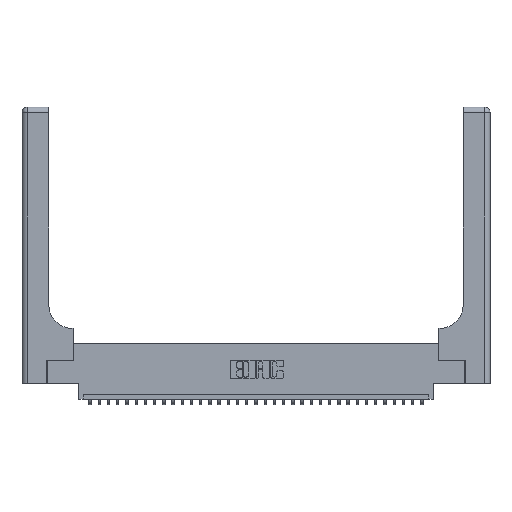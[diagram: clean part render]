
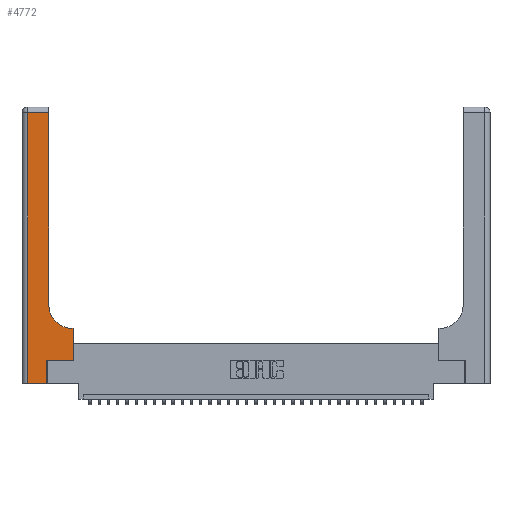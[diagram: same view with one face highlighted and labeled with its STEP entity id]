
A CAD part, top view. The second image highlights one B-rep face of the part: STEP entity #4772.
In plain terms, the highlighted planar face has unit normal (0, 0, 1).
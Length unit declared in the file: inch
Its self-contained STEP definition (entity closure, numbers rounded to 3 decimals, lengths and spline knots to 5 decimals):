
#44 = ORIENTED_EDGE ( 'NONE', *, *, #14090, .T. ) ;
#90 = AXIS2_PLACEMENT_3D ( 'NONE', #28757, #23388, #31163 ) ;
#210 = EDGE_CURVE ( 'NONE', #9094, #18369, #2302, .T. ) ;
#409 = CARTESIAN_POINT ( 'NONE',  ( 0.269, 0.25, 0.37 ) ) ;
#1232 = ORIENTED_EDGE ( 'NONE', *, *, #210, .T. ) ;
#1958 = DIRECTION ( 'NONE',  ( 0., 0., -1. ) ) ;
#2302 = LINE ( 'NONE', #22359, #29274 ) ;
#2518 = VERTEX_POINT ( 'NONE', #10533 ) ;
#2566 = DIRECTION ( 'NONE',  ( -1., 0., 0. ) ) ;
#2867 = ORIENTED_EDGE ( 'NONE', *, *, #11220, .T. ) ;
#3113 = EDGE_LOOP ( 'NONE', ( #7505, #2867, #10119, #4318, #21467, #23054, #8363, #1232, #44 ) ) ;
#3126 = CARTESIAN_POINT ( 'NONE',  ( 0.269, 0., 0.37 ) ) ;
#4318 = ORIENTED_EDGE ( 'NONE', *, *, #21432, .T. ) ;
#4324 = VECTOR ( 'NONE', #20826, 39.37008 ) ;
#4772 = ADVANCED_FACE ( 'NONE', ( #20979 ), #33293, .F. ) ;
#5705 = VERTEX_POINT ( 'NONE', #21931 ) ;
#5923 = CARTESIAN_POINT ( 'NONE',  ( 0., 0., 0.37 ) ) ;
#6923 = LINE ( 'NONE', #29094, #13025 ) ;
#7229 = LINE ( 'NONE', #25717, #4324 ) ;
#7505 = ORIENTED_EDGE ( 'NONE', *, *, #13925, .T. ) ;
#7593 = VECTOR ( 'NONE', #12002, 39.37008 ) ;
#8363 = ORIENTED_EDGE ( 'NONE', *, *, #13276, .T. ) ;
#9094 = VERTEX_POINT ( 'NONE', #18933 ) ;
#9532 = CARTESIAN_POINT ( 'NONE',  ( 0., 3., 0.37 ) ) ;
#9548 = EDGE_CURVE ( 'NONE', #2518, #12642, #27146, .T. ) ;
#9714 = VECTOR ( 'NONE', #29670, 39.37008 ) ;
#9874 = DIRECTION ( 'NONE',  ( -1., 0., 0. ) ) ;
#10119 = ORIENTED_EDGE ( 'NONE', *, *, #9548, .T. ) ;
#10533 = CARTESIAN_POINT ( 'NONE',  ( 0.06, 2.94, 0.37 ) ) ;
#11220 = EDGE_CURVE ( 'NONE', #16328, #2518, #6923, .T. ) ;
#12002 = DIRECTION ( 'NONE',  ( 0., 1., 0. ) ) ;
#12408 = DIRECTION ( 'NONE',  ( -1., 0., 0. ) ) ;
#12642 = VERTEX_POINT ( 'NONE', #25406 ) ;
#13025 = VECTOR ( 'NONE', #12408, 39.37008 ) ;
#13276 = EDGE_CURVE ( 'NONE', #19494, #9094, #7229, .T. ) ;
#13925 = EDGE_CURVE ( 'NONE', #20428, #16328, #26750, .T. ) ;
#14090 = EDGE_CURVE ( 'NONE', #18369, #20428, #29173, .T. ) ;
#16266 = CARTESIAN_POINT ( 'NONE',  ( 0.5585, 0.25, 0.37 ) ) ;
#16328 = VERTEX_POINT ( 'NONE', #25529 ) ;
#17271 = CARTESIAN_POINT ( 'NONE',  ( 0.5415, 0.6, 0.37 ) ) ;
#18067 = VECTOR ( 'NONE', #24955, 39.37008 ) ;
#18369 = VERTEX_POINT ( 'NONE', #17271 ) ;
#18705 = EDGE_CURVE ( 'NONE', #5705, #31359, #28296, .T. ) ;
#18933 = CARTESIAN_POINT ( 'NONE',  ( 0.5585, 0.6, 0.37 ) ) ;
#19494 = VERTEX_POINT ( 'NONE', #16266 ) ;
#20114 = AXIS2_PLACEMENT_3D ( 'NONE', #9532, #1958, #9874 ) ;
#20218 = DIRECTION ( 'NONE',  ( 0., -1., 0. ) ) ;
#20428 = VERTEX_POINT ( 'NONE', #23429 ) ;
#20826 = DIRECTION ( 'NONE',  ( 0., 1., 0. ) ) ;
#20979 = FACE_OUTER_BOUND ( 'NONE', #3113, .T. ) ;
#21432 = EDGE_CURVE ( 'NONE', #12642, #5705, #29283, .T. ) ;
#21467 = ORIENTED_EDGE ( 'NONE', *, *, #18705, .T. ) ;
#21682 = CARTESIAN_POINT ( 'NONE',  ( 0.269, 0.25, 0.37 ) ) ;
#21931 = CARTESIAN_POINT ( 'NONE',  ( 0.269, 0., 0.37 ) ) ;
#22359 = CARTESIAN_POINT ( 'NONE',  ( 0.2915, 0.6, 0.37 ) ) ;
#23054 = ORIENTED_EDGE ( 'NONE', *, *, #30145, .T. ) ;
#23388 = DIRECTION ( 'NONE',  ( 0., 0., -1. ) ) ;
#23429 = CARTESIAN_POINT ( 'NONE',  ( 0.2915, 0.85, 0.37 ) ) ;
#24955 = DIRECTION ( 'NONE',  ( 0., 1., 0. ) ) ;
#25406 = CARTESIAN_POINT ( 'NONE',  ( 0.06, 0., 0.37 ) ) ;
#25529 = CARTESIAN_POINT ( 'NONE',  ( 0.2915, 2.94, 0.37 ) ) ;
#25717 = CARTESIAN_POINT ( 'NONE',  ( 0.5585, 0.25, 0.37 ) ) ;
#26750 = LINE ( 'NONE', #27663, #7593 ) ;
#27146 = LINE ( 'NONE', #33370, #33291 ) ;
#27663 = CARTESIAN_POINT ( 'NONE',  ( 0.2915, 3., 0.37 ) ) ;
#28296 = LINE ( 'NONE', #3126, #18067 ) ;
#28757 = CARTESIAN_POINT ( 'NONE',  ( 0.5415, 0.85, 0.37 ) ) ;
#29094 = CARTESIAN_POINT ( 'NONE',  ( 0., 2.94, 0.37 ) ) ;
#29173 = CIRCLE ( 'NONE', #90, 0.25 ) ;
#29274 = VECTOR ( 'NONE', #2566, 39.37008 ) ;
#29283 = LINE ( 'NONE', #5923, #9714 ) ;
#29670 = DIRECTION ( 'NONE',  ( 1., 0., 0. ) ) ;
#29907 = DIRECTION ( 'NONE',  ( 1., 0., 0. ) ) ;
#30145 = EDGE_CURVE ( 'NONE', #31359, #19494, #32570, .T. ) ;
#31163 = DIRECTION ( 'NONE',  ( 1., 0., 0. ) ) ;
#31359 = VERTEX_POINT ( 'NONE', #409 ) ;
#31696 = VECTOR ( 'NONE', #29907, 39.37008 ) ;
#32570 = LINE ( 'NONE', #21682, #31696 ) ;
#33291 = VECTOR ( 'NONE', #20218, 39.37008 ) ;
#33293 = PLANE ( 'NONE',  #20114 ) ;
#33370 = CARTESIAN_POINT ( 'NONE',  ( 0.06, 3., 0.37 ) ) ;
